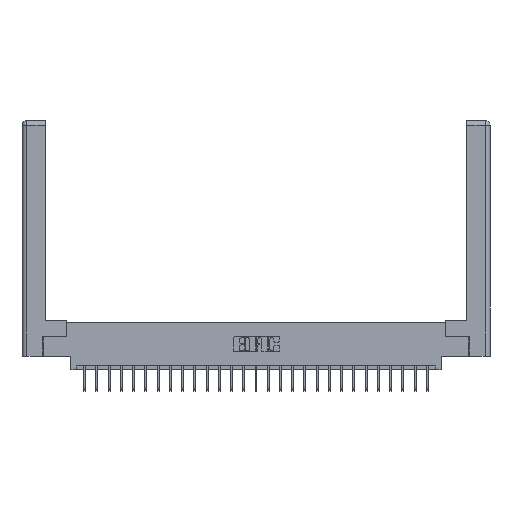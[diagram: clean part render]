
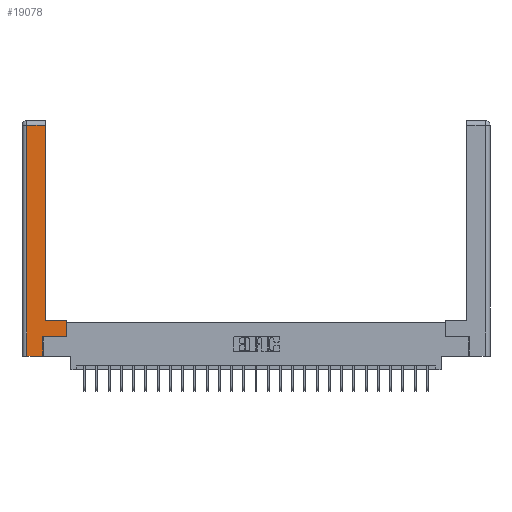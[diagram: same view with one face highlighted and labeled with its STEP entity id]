
A CAD part, top view. The second image highlights one B-rep face of the part: STEP entity #19078.
In plain terms, the highlighted planar face has unit normal (0, 0, 1).
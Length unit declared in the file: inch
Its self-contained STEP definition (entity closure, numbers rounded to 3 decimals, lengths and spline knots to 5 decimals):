
#661 = LINE ( 'NONE', #21755, #23605 ) ;
#1034 = EDGE_CURVE ( 'NONE', #19639, #3407, #6197, .T. ) ;
#2430 = VERTEX_POINT ( 'NONE', #17282 ) ;
#2475 = VECTOR ( 'NONE', #28748, 39.37008 ) ;
#3043 = ORIENTED_EDGE ( 'NONE', *, *, #8301, .T. ) ;
#3407 = VERTEX_POINT ( 'NONE', #26229 ) ;
#3617 = ORIENTED_EDGE ( 'NONE', *, *, #28445, .T. ) ;
#4413 = CARTESIAN_POINT ( 'NONE',  ( 0.295, 0.45, 0. ) ) ;
#5164 = CARTESIAN_POINT ( 'NONE',  ( 0.295, 0.45, 0. ) ) ;
#5357 = VECTOR ( 'NONE', #20032, 39.37008 ) ;
#5730 = EDGE_CURVE ( 'NONE', #9067, #16963, #21857, .T. ) ;
#5846 = ORIENTED_EDGE ( 'NONE', *, *, #1034, .T. ) ;
#6197 = LINE ( 'NONE', #15877, #22195 ) ;
#6567 = VECTOR ( 'NONE', #27454, 39.37008 ) ;
#8187 = VERTEX_POINT ( 'NONE', #5164 ) ;
#8301 = EDGE_CURVE ( 'NONE', #3407, #27377, #10927, .T. ) ;
#8516 = EDGE_CURVE ( 'NONE', #25072, #19639, #8857, .T. ) ;
#8857 = LINE ( 'NONE', #15648, #5357 ) ;
#9067 = VERTEX_POINT ( 'NONE', #15004 ) ;
#9626 = CARTESIAN_POINT ( 'NONE',  ( 0.265, 0., 0. ) ) ;
#9946 = ORIENTED_EDGE ( 'NONE', *, *, #8516, .T. ) ;
#10481 = PLANE ( 'NONE',  #16435 ) ;
#10517 = CARTESIAN_POINT ( 'NONE',  ( 0.265, 0.245, 0. ) ) ;
#10575 = CARTESIAN_POINT ( 'NONE',  ( 0., 0., 0. ) ) ;
#10927 = LINE ( 'NONE', #18821, #17920 ) ;
#11135 = LINE ( 'NONE', #16496, #27403 ) ;
#11546 = CARTESIAN_POINT ( 'NONE',  ( 0.0615, 2.94, 0. ) ) ;
#11858 = LINE ( 'NONE', #9626, #6567 ) ;
#14034 = LINE ( 'NONE', #4413, #2475 ) ;
#14377 = DIRECTION ( 'NONE',  ( 0., 1., 0. ) ) ;
#15004 = CARTESIAN_POINT ( 'NONE',  ( 0.295, 2.94, 0. ) ) ;
#15528 = DIRECTION ( 'NONE',  ( 0., 1., 0. ) ) ;
#15648 = CARTESIAN_POINT ( 'NONE',  ( 0.265, 0.245, 0. ) ) ;
#15877 = CARTESIAN_POINT ( 'NONE',  ( 0.565, 0.245, 0. ) ) ;
#16435 = AXIS2_PLACEMENT_3D ( 'NONE', #10575, #17601, #26404 ) ;
#16496 = CARTESIAN_POINT ( 'NONE',  ( 0.0615, 0., 0. ) ) ;
#16550 = ORIENTED_EDGE ( 'NONE', *, *, #5730, .T. ) ;
#16963 = VERTEX_POINT ( 'NONE', #11546 ) ;
#17282 = CARTESIAN_POINT ( 'NONE',  ( 0.0615, 0., 0. ) ) ;
#17601 = DIRECTION ( 'NONE',  ( 0., 0., -1. ) ) ;
#17700 = EDGE_LOOP ( 'NONE', ( #24304, #16550, #25050, #22848, #9946, #5846, #3043, #3617 ) ) ;
#17920 = VECTOR ( 'NONE', #14377, 39.37008 ) ;
#18821 = CARTESIAN_POINT ( 'NONE',  ( 0.565, 0.45, 0. ) ) ;
#19078 = ADVANCED_FACE ( 'NONE', ( #22266 ), #10481, .F. ) ;
#19384 = DIRECTION ( 'NONE',  ( -1., 0., 0. ) ) ;
#19639 = VERTEX_POINT ( 'NONE', #10517 ) ;
#19792 = EDGE_CURVE ( 'NONE', #8187, #9067, #661, .T. ) ;
#20032 = DIRECTION ( 'NONE',  ( 0., 1., 0. ) ) ;
#21394 = CARTESIAN_POINT ( 'NONE',  ( 0.0615, 2.94, 0. ) ) ;
#21755 = CARTESIAN_POINT ( 'NONE',  ( 0.295, 3., 0. ) ) ;
#21857 = LINE ( 'NONE', #21394, #22531 ) ;
#22195 = VECTOR ( 'NONE', #25704, 39.37008 ) ;
#22241 = CARTESIAN_POINT ( 'NONE',  ( 0.265, 0., 0. ) ) ;
#22266 = FACE_OUTER_BOUND ( 'NONE', #17700, .T. ) ;
#22531 = VECTOR ( 'NONE', #19384, 39.37008 ) ;
#22848 = ORIENTED_EDGE ( 'NONE', *, *, #25799, .T. ) ;
#23099 = DIRECTION ( 'NONE',  ( 0., -1., 0. ) ) ;
#23605 = VECTOR ( 'NONE', #15528, 39.37008 ) ;
#24304 = ORIENTED_EDGE ( 'NONE', *, *, #19792, .T. ) ;
#25050 = ORIENTED_EDGE ( 'NONE', *, *, #25831, .T. ) ;
#25072 = VERTEX_POINT ( 'NONE', #22241 ) ;
#25704 = DIRECTION ( 'NONE',  ( 1., 0., 0. ) ) ;
#25799 = EDGE_CURVE ( 'NONE', #2430, #25072, #11858, .T. ) ;
#25831 = EDGE_CURVE ( 'NONE', #16963, #2430, #11135, .T. ) ;
#26229 = CARTESIAN_POINT ( 'NONE',  ( 0.565, 0.245, 0. ) ) ;
#26404 = DIRECTION ( 'NONE',  ( -1., 0., 0. ) ) ;
#27146 = CARTESIAN_POINT ( 'NONE',  ( 0.565, 0.45, 0. ) ) ;
#27377 = VERTEX_POINT ( 'NONE', #27146 ) ;
#27403 = VECTOR ( 'NONE', #23099, 39.37008 ) ;
#27454 = DIRECTION ( 'NONE',  ( 1., 0., 0. ) ) ;
#28445 = EDGE_CURVE ( 'NONE', #27377, #8187, #14034, .T. ) ;
#28748 = DIRECTION ( 'NONE',  ( -1., 0., 0. ) ) ;
